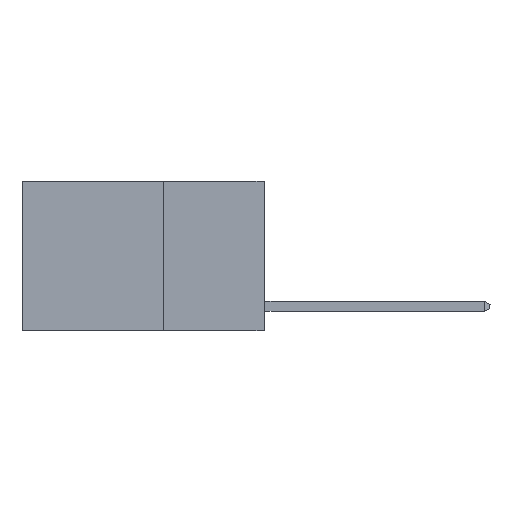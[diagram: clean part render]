
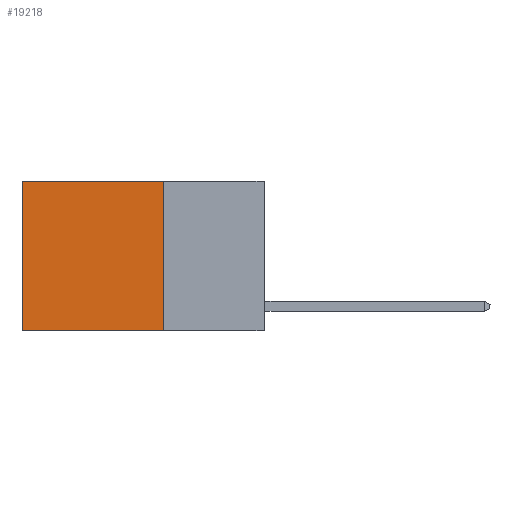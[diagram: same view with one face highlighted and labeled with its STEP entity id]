
A CAD part, left-side view. The second image highlights one B-rep face of the part: STEP entity #19218.
In plain terms, the highlighted planar face has unit normal (-1, 0, 0).
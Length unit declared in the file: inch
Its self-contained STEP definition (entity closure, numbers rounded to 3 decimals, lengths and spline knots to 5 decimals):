
#148 = LINE ( 'NONE', #9640, #11794 ) ;
#1169 = VERTEX_POINT ( 'NONE', #7460 ) ;
#1578 = ORIENTED_EDGE ( 'NONE', *, *, #6403, .T. ) ;
#2232 = CARTESIAN_POINT ( 'NONE',  ( 0.2625, 0.25, 0. ) ) ;
#3556 = ORIENTED_EDGE ( 'NONE', *, *, #16353, .T. ) ;
#4216 = VECTOR ( 'NONE', #7015, 39.37008 ) ;
#4479 = EDGE_CURVE ( 'NONE', #1169, #14024, #11862, .T. ) ;
#4722 = CARTESIAN_POINT ( 'NONE',  ( 0.2625, 0.6, 0. ) ) ;
#6403 = EDGE_CURVE ( 'NONE', #13432, #9725, #8721, .T. ) ;
#7015 = DIRECTION ( 'NONE',  ( 0., 0., -1. ) ) ;
#7368 = PLANE ( 'NONE',  #16012 ) ;
#7460 = CARTESIAN_POINT ( 'NONE',  ( 0.2625, 0.25, 0. ) ) ;
#7862 = EDGE_LOOP ( 'NONE', ( #1578, #13108, #9492, #3556 ) ) ;
#8721 = LINE ( 'NONE', #14503, #4216 ) ;
#8898 = DIRECTION ( 'NONE',  ( 1., 0., 0. ) ) ;
#9492 = ORIENTED_EDGE ( 'NONE', *, *, #4479, .F. ) ;
#9640 = CARTESIAN_POINT ( 'NONE',  ( 0.2625, 0.25, 0. ) ) ;
#9725 = VERTEX_POINT ( 'NONE', #11547 ) ;
#11547 = CARTESIAN_POINT ( 'NONE',  ( 0.2625, 0.6, -0.37 ) ) ;
#11794 = VECTOR ( 'NONE', #14069, 39.37008 ) ;
#11862 = LINE ( 'NONE', #2232, #15831 ) ;
#12015 = VECTOR ( 'NONE', #17571, 39.37008 ) ;
#12140 = CARTESIAN_POINT ( 'NONE',  ( 0.2625, 0.25, -0.37 ) ) ;
#12796 = DIRECTION ( 'NONE',  ( 0., 0., -1. ) ) ;
#13108 = ORIENTED_EDGE ( 'NONE', *, *, #16566, .F. ) ;
#13432 = VERTEX_POINT ( 'NONE', #4722 ) ;
#14024 = VERTEX_POINT ( 'NONE', #12140 ) ;
#14069 = DIRECTION ( 'NONE',  ( 0., 1., 0. ) ) ;
#14503 = CARTESIAN_POINT ( 'NONE',  ( 0.2625, 0.6, 0. ) ) ;
#15831 = VECTOR ( 'NONE', #12796, 39.37008 ) ;
#15998 = LINE ( 'NONE', #16120, #12015 ) ;
#16012 = AXIS2_PLACEMENT_3D ( 'NONE', #17828, #8898, #19315 ) ;
#16120 = CARTESIAN_POINT ( 'NONE',  ( 0.2625, 0.25, -0.37 ) ) ;
#16353 = EDGE_CURVE ( 'NONE', #1169, #13432, #148, .T. ) ;
#16566 = EDGE_CURVE ( 'NONE', #14024, #9725, #15998, .T. ) ;
#17571 = DIRECTION ( 'NONE',  ( 0., 1., 0. ) ) ;
#17828 = CARTESIAN_POINT ( 'NONE',  ( 0.2625, 0.25, 0. ) ) ;
#18643 = FACE_OUTER_BOUND ( 'NONE', #7862, .T. ) ;
#19218 = ADVANCED_FACE ( 'NONE', ( #18643 ), #7368, .F. ) ;
#19315 = DIRECTION ( 'NONE',  ( 0., 0., -1. ) ) ;
